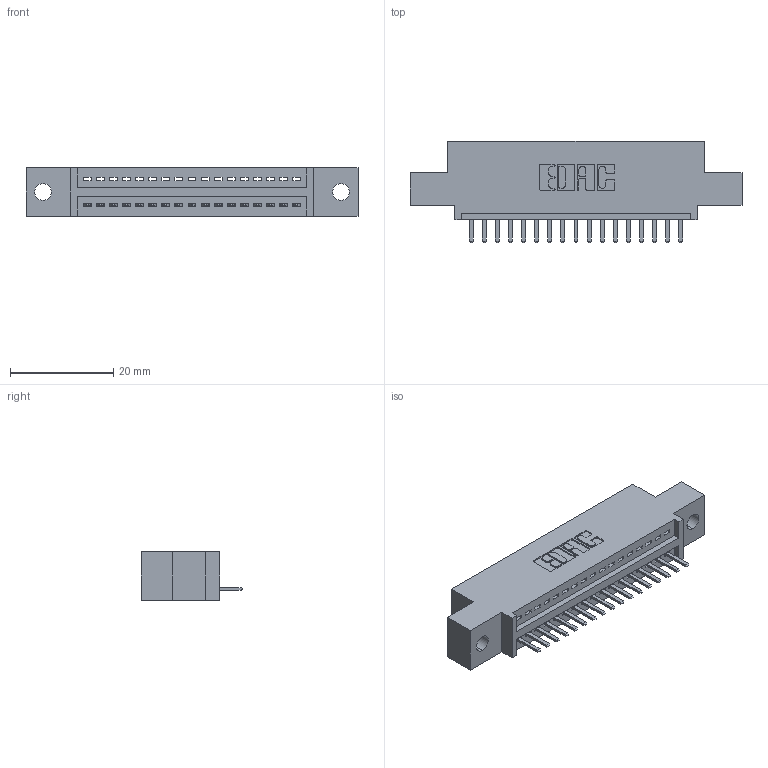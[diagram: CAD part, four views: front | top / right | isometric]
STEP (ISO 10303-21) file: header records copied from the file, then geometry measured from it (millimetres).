
FILE_DESCRIPTION (( 'STEP AP203' ), '1' );
FILE_NAME ('395-017-520-402.STEP', '2019-10-17T13:56:59', ( '' ), ( '' ), 'SwSTEP 2.0', 'SolidWorks 2016', '' );
FILE_SCHEMA (( 'CONFIG_CONTROL_DESIGN' ));
Length unit declared in the file: inch
Products named in the file (3): 395-017-520-402; 345-292-001_345-293-120; 345 Part_0.110 Offset - 0.128 Dia
Assembly tree (18 placements, depth 2):
  395-017-520-402
    345 Part_0.110 Offset - 0.128 Dia
    345-292-001_345-293-120  x17
Bounding box: 64.39 x 19.68 x 9.4 mm (x, y, z)
Volume: 5752 mm3; surface area: 6954.5 mm2
Topology: 18 solids, 18 shells, 1184 faces, 3481 edges, 2274 vertices
Faces by surface type: plane 798, cylinder 386
Entity records: 16409 total; most frequent: CARTESIAN_POINT 2863, ORIENTED_EDGE 2802, DIRECTION 2523, EDGE_CURVE 1401, LINE 1197, VECTOR 1197, VERTEX_POINT 930, AXIS2_PLACEMENT_3D 663
